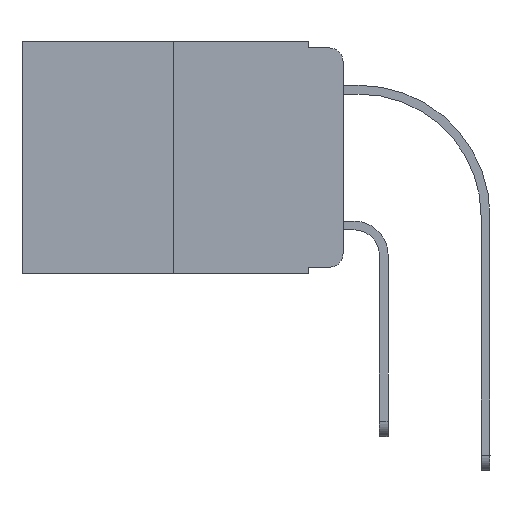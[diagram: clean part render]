
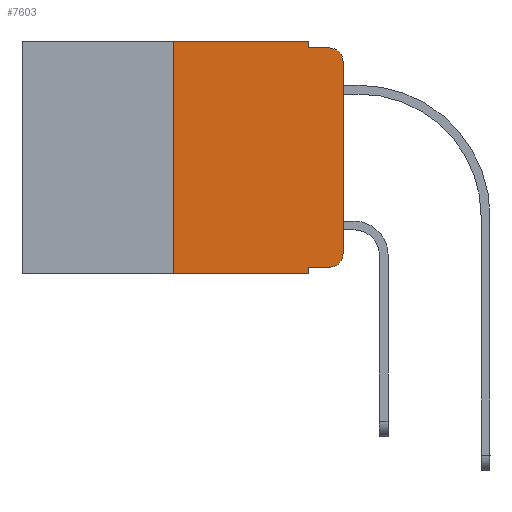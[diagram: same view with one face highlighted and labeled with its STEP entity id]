
A CAD part, left-side view. The second image highlights one B-rep face of the part: STEP entity #7603.
In plain terms, the highlighted planar face has unit normal (-1, 0, 0).
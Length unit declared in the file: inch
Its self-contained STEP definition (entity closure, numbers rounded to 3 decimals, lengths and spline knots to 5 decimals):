
#62 = FACE_OUTER_BOUND ( 'NONE', #18552, .T. ) ;
#392 = EDGE_CURVE ( 'NONE', #23397, #16810, #3510, .T. ) ;
#509 = VERTEX_POINT ( 'NONE', #15708 ) ;
#602 = ORIENTED_EDGE ( 'NONE', *, *, #3079, .F. ) ;
#1669 = AXIS2_PLACEMENT_3D ( 'NONE', #7069, #12570, #5223 ) ;
#1873 = DIRECTION ( 'NONE',  ( 0., -1., 0. ) ) ;
#1963 = CARTESIAN_POINT ( 'NONE',  ( 0., 0.051, -0.343 ) ) ;
#2062 = DIRECTION ( 'NONE',  ( 1., 0., 0. ) ) ;
#2180 = CARTESIAN_POINT ( 'NONE',  ( 0., 0.051, 0. ) ) ;
#2408 = ORIENTED_EDGE ( 'NONE', *, *, #5576, .T. ) ;
#2568 = VECTOR ( 'NONE', #19763, 39.37008 ) ;
#2712 = ORIENTED_EDGE ( 'NONE', *, *, #392, .T. ) ;
#2914 = CARTESIAN_POINT ( 'NONE',  ( 0., 0.25, 0. ) ) ;
#3079 = EDGE_CURVE ( 'NONE', #5471, #8132, #6771, .T. ) ;
#3510 = LINE ( 'NONE', #18732, #20631 ) ;
#3921 = PLANE ( 'NONE',  #11854 ) ;
#5223 = DIRECTION ( 'NONE',  ( 0., 0., -1. ) ) ;
#5471 = VERTEX_POINT ( 'NONE', #18322 ) ;
#5576 = EDGE_CURVE ( 'NONE', #17842, #23397, #15994, .T. ) ;
#6771 = LINE ( 'NONE', #20017, #16232 ) ;
#6934 = EDGE_CURVE ( 'NONE', #15122, #13770, #16221, .T. ) ;
#7069 = CARTESIAN_POINT ( 'NONE',  ( 0., 0.02, -0.313 ) ) ;
#7371 = CARTESIAN_POINT ( 'NONE',  ( 0., 0.473, -0.343 ) ) ;
#7603 = ADVANCED_FACE ( 'NONE', ( #62 ), #3921, .F. ) ;
#7686 = DIRECTION ( 'NONE',  ( -1., 0., 0. ) ) ;
#7838 = CARTESIAN_POINT ( 'NONE',  ( 0., 0.02, -0.333 ) ) ;
#7922 = VECTOR ( 'NONE', #12232, 39.37008 ) ;
#8132 = VERTEX_POINT ( 'NONE', #2914 ) ;
#8166 = EDGE_CURVE ( 'NONE', #5471, #13770, #14963, .T. ) ;
#8636 = CARTESIAN_POINT ( 'NONE',  ( 0., 0.473, 0. ) ) ;
#8724 = VERTEX_POINT ( 'NONE', #24582 ) ;
#9225 = ORIENTED_EDGE ( 'NONE', *, *, #8166, .T. ) ;
#9663 = DIRECTION ( 'NONE',  ( 0., 0., -1. ) ) ;
#9909 = EDGE_CURVE ( 'NONE', #16810, #509, #21676, .T. ) ;
#10093 = CARTESIAN_POINT ( 'NONE',  ( 0., 0.051, -0.01 ) ) ;
#10146 = LINE ( 'NONE', #8636, #2568 ) ;
#10381 = VECTOR ( 'NONE', #22950, 39.37008 ) ;
#10483 = EDGE_CURVE ( 'NONE', #8132, #8724, #10146, .T. ) ;
#10572 = EDGE_CURVE ( 'NONE', #15122, #17842, #22495, .T. ) ;
#11336 = ORIENTED_EDGE ( 'NONE', *, *, #9909, .T. ) ;
#11519 = CARTESIAN_POINT ( 'NONE',  ( 0., 0.473, 0. ) ) ;
#11669 = DIRECTION ( 'NONE',  ( 0., 0., -1. ) ) ;
#11854 = AXIS2_PLACEMENT_3D ( 'NONE', #11519, #2062, #9663 ) ;
#12232 = DIRECTION ( 'NONE',  ( 0., 0., -1. ) ) ;
#12390 = VERTEX_POINT ( 'NONE', #13874 ) ;
#12488 = EDGE_CURVE ( 'NONE', #8724, #12390, #19270, .T. ) ;
#12512 = VECTOR ( 'NONE', #24017, 39.37008 ) ;
#12570 = DIRECTION ( 'NONE',  ( -1., 0., 0. ) ) ;
#13016 = VECTOR ( 'NONE', #1873, 39.37008 ) ;
#13284 = EDGE_CURVE ( 'NONE', #12390, #509, #23211, .T. ) ;
#13342 = DIRECTION ( 'NONE',  ( 0., 0., 1. ) ) ;
#13406 = CARTESIAN_POINT ( 'NONE',  ( 0., 0.02, -0.03 ) ) ;
#13770 = VERTEX_POINT ( 'NONE', #1963 ) ;
#13874 = CARTESIAN_POINT ( 'NONE',  ( 0., 0.051, -0.01 ) ) ;
#14963 = LINE ( 'NONE', #7371, #13016 ) ;
#15122 = VERTEX_POINT ( 'NONE', #21047 ) ;
#15277 = AXIS2_PLACEMENT_3D ( 'NONE', #13406, #7686, #11669 ) ;
#15708 = CARTESIAN_POINT ( 'NONE',  ( 0., 0.02, -0.01 ) ) ;
#15994 = CIRCLE ( 'NONE', #1669, 0.02 ) ;
#16100 = CARTESIAN_POINT ( 'NONE',  ( 0., 0., -0.313 ) ) ;
#16221 = LINE ( 'NONE', #23615, #7922 ) ;
#16232 = VECTOR ( 'NONE', #20246, 39.37008 ) ;
#16501 = CARTESIAN_POINT ( 'NONE',  ( 0., 0.051, -0.333 ) ) ;
#16810 = VERTEX_POINT ( 'NONE', #20420 ) ;
#17006 = ORIENTED_EDGE ( 'NONE', *, *, #13284, .F. ) ;
#17371 = ORIENTED_EDGE ( 'NONE', *, *, #10483, .F. ) ;
#17389 = DIRECTION ( 'NONE',  ( 0., 0., -1. ) ) ;
#17842 = VERTEX_POINT ( 'NONE', #7838 ) ;
#18322 = CARTESIAN_POINT ( 'NONE',  ( 0., 0.25, -0.343 ) ) ;
#18552 = EDGE_LOOP ( 'NONE', ( #2712, #11336, #17006, #20439, #17371, #602, #9225, #22393, #19630, #2408 ) ) ;
#18732 = CARTESIAN_POINT ( 'NONE',  ( 0., 0., 0. ) ) ;
#19270 = LINE ( 'NONE', #2180, #19915 ) ;
#19630 = ORIENTED_EDGE ( 'NONE', *, *, #10572, .T. ) ;
#19763 = DIRECTION ( 'NONE',  ( 0., -1., 0. ) ) ;
#19915 = VECTOR ( 'NONE', #17389, 39.37008 ) ;
#20017 = CARTESIAN_POINT ( 'NONE',  ( 0., 0.25, 0. ) ) ;
#20246 = DIRECTION ( 'NONE',  ( 0., 0., 1. ) ) ;
#20420 = CARTESIAN_POINT ( 'NONE',  ( 0., 0., -0.03 ) ) ;
#20439 = ORIENTED_EDGE ( 'NONE', *, *, #12488, .F. ) ;
#20631 = VECTOR ( 'NONE', #13342, 39.37008 ) ;
#21047 = CARTESIAN_POINT ( 'NONE',  ( 0., 0.051, -0.333 ) ) ;
#21676 = CIRCLE ( 'NONE', #15277, 0.02 ) ;
#22393 = ORIENTED_EDGE ( 'NONE', *, *, #6934, .F. ) ;
#22495 = LINE ( 'NONE', #16501, #12512 ) ;
#22950 = DIRECTION ( 'NONE',  ( 0., -1., 0. ) ) ;
#23211 = LINE ( 'NONE', #10093, #10381 ) ;
#23397 = VERTEX_POINT ( 'NONE', #16100 ) ;
#23615 = CARTESIAN_POINT ( 'NONE',  ( 0., 0.051, 0. ) ) ;
#24017 = DIRECTION ( 'NONE',  ( 0., -1., 0. ) ) ;
#24582 = CARTESIAN_POINT ( 'NONE',  ( 0., 0.051, 0. ) ) ;
